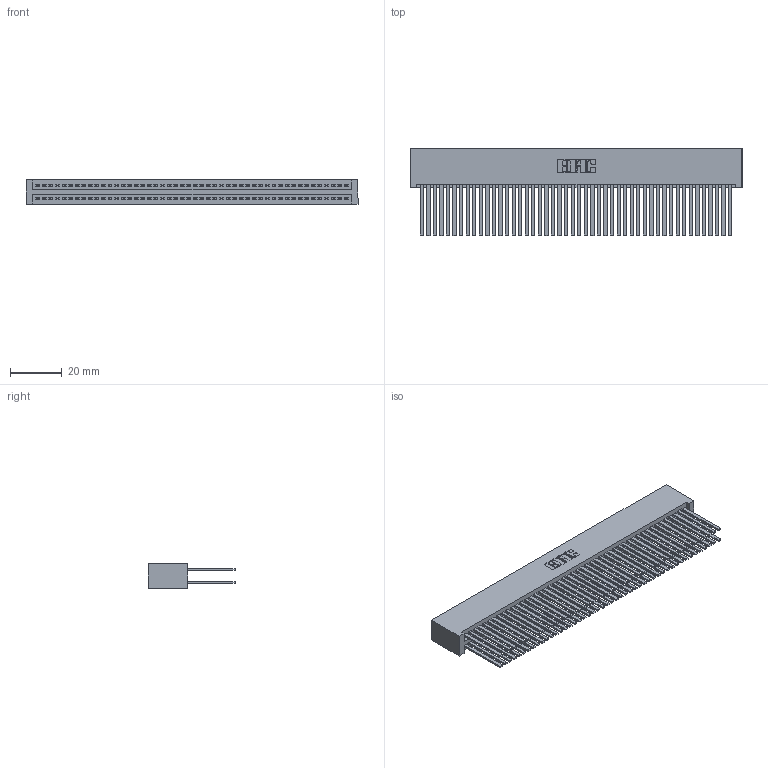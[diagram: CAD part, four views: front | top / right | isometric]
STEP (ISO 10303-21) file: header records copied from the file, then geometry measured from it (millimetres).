
FILE_DESCRIPTION (( 'STEP AP203' ), '1' );
FILE_NAME ('395-096-544-201.STEP', '2018-11-29T16:17:31', ( '' ), ( '' ), 'SwSTEP 2.0', 'SolidWorks 2016', '' );
FILE_SCHEMA (( 'CONFIG_CONTROL_DESIGN' ));
Length unit declared in the file: inch
Products named in the file (3): 345-292-001_345-293-144; 345 Part_No Mounting Lugs; 395-096-544-201
Assembly tree (97 placements, depth 2):
  395-096-544-201
    345 Part_No Mounting Lugs
    345-292-001_345-293-144  x96
Bounding box: 128.52 x 33.96 x 9.4 mm (x, y, z)
Volume: 14502.3 mm3; surface area: 25800.6 mm2
Topology: 97 solids, 97 shells, 4342 faces, 12893 edges, 8466 vertices
Faces by surface type: plane 2860, cylinder 1482
Entity records: 36393 total; most frequent: CARTESIAN_POINT 6092, ORIENTED_EDGE 6026, DIRECTION 5357, EDGE_CURVE 3013, VECTOR 2701, LINE 2701, VERTEX_POINT 2006, AXIS2_PLACEMENT_3D 1328
